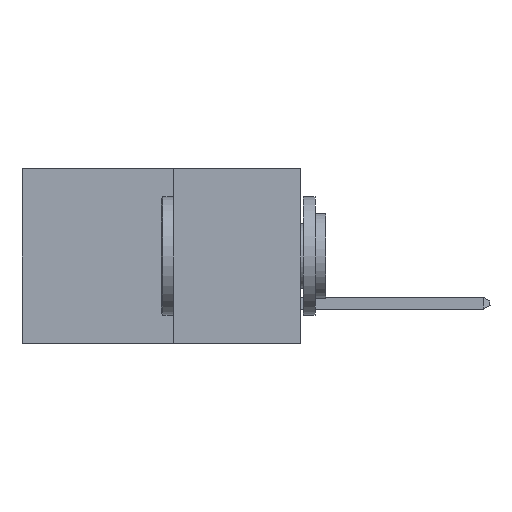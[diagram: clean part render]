
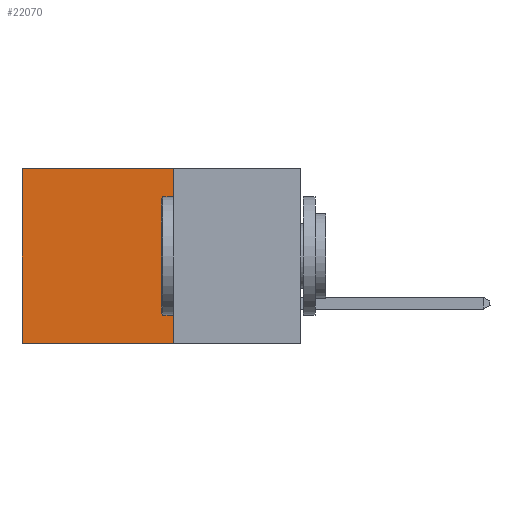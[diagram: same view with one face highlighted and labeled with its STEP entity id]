
A CAD part, left-side view. The second image highlights one B-rep face of the part: STEP entity #22070.
In plain terms, the highlighted planar face has unit normal (-1, 0, 0).
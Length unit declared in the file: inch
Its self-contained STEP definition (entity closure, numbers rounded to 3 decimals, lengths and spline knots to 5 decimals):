
#1314 = EDGE_CURVE ( 'NONE', #6254, #7374, #3422, .T. ) ;
#2283 = ORIENTED_EDGE ( 'NONE', *, *, #1314, .T. ) ;
#2776 = EDGE_LOOP ( 'NONE', ( #2283, #3388, #20356, #10017 ) ) ;
#3388 = ORIENTED_EDGE ( 'NONE', *, *, #14891, .F. ) ;
#3392 = CARTESIAN_POINT ( 'NONE',  ( 0.277, 0.59, -0.37 ) ) ;
#3422 = LINE ( 'NONE', #11504, #18835 ) ;
#4376 = DIRECTION ( 'NONE',  ( 0., 1., 0. ) ) ;
#5202 = VERTEX_POINT ( 'NONE', #5659 ) ;
#5443 = EDGE_CURVE ( 'NONE', #5202, #15010, #17829, .T. ) ;
#5659 = CARTESIAN_POINT ( 'NONE',  ( 0.277, 0.27, 0. ) ) ;
#6057 = CARTESIAN_POINT ( 'NONE',  ( 0.277, 0.27, 0. ) ) ;
#6254 = VERTEX_POINT ( 'NONE', #14266 ) ;
#7374 = VERTEX_POINT ( 'NONE', #3392 ) ;
#8433 = PLANE ( 'NONE',  #17203 ) ;
#8667 = VECTOR ( 'NONE', #22004, 39.37008 ) ;
#9328 = LINE ( 'NONE', #6057, #21738 ) ;
#9879 = CARTESIAN_POINT ( 'NONE',  ( 0.277, 0.27, -0.37 ) ) ;
#10017 = ORIENTED_EDGE ( 'NONE', *, *, #14750, .T. ) ;
#10088 = CARTESIAN_POINT ( 'NONE',  ( 0.277, 0.27, -0.37 ) ) ;
#10153 = DIRECTION ( 'NONE',  ( 0., 0., -1. ) ) ;
#10174 = CARTESIAN_POINT ( 'NONE',  ( 0.277, 0.27, -0.37 ) ) ;
#10676 = VECTOR ( 'NONE', #11621, 39.37008 ) ;
#11504 = CARTESIAN_POINT ( 'NONE',  ( 0.277, 0.59, -0.37 ) ) ;
#11621 = DIRECTION ( 'NONE',  ( 0., 1., 0. ) ) ;
#14266 = CARTESIAN_POINT ( 'NONE',  ( 0.277, 0.59, 0. ) ) ;
#14750 = EDGE_CURVE ( 'NONE', #5202, #6254, #9328, .T. ) ;
#14891 = EDGE_CURVE ( 'NONE', #15010, #7374, #19818, .T. ) ;
#15010 = VERTEX_POINT ( 'NONE', #10174 ) ;
#15871 = FACE_OUTER_BOUND ( 'NONE', #2776, .T. ) ;
#17203 = AXIS2_PLACEMENT_3D ( 'NONE', #10088, #20398, #10153 ) ;
#17829 = LINE ( 'NONE', #22060, #8667 ) ;
#18835 = VECTOR ( 'NONE', #19534, 39.37008 ) ;
#19534 = DIRECTION ( 'NONE',  ( 0., 0., -1. ) ) ;
#19818 = LINE ( 'NONE', #9879, #10676 ) ;
#20356 = ORIENTED_EDGE ( 'NONE', *, *, #5443, .F. ) ;
#20398 = DIRECTION ( 'NONE',  ( 1., 0., 0. ) ) ;
#21738 = VECTOR ( 'NONE', #4376, 39.37008 ) ;
#22004 = DIRECTION ( 'NONE',  ( 0., 0., -1. ) ) ;
#22060 = CARTESIAN_POINT ( 'NONE',  ( 0.277, 0.27, -0.37 ) ) ;
#22070 = ADVANCED_FACE ( 'NONE', ( #15871 ), #8433, .F. ) ;
